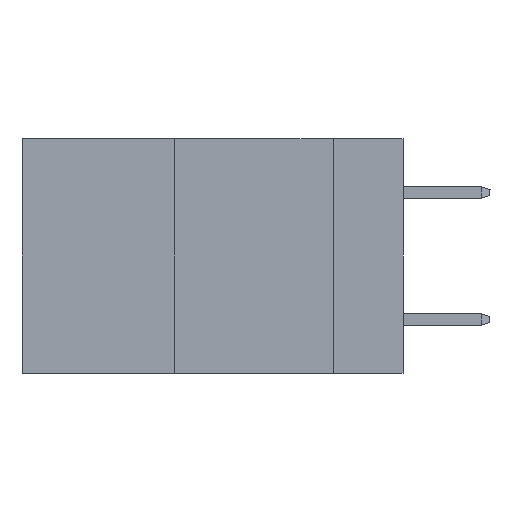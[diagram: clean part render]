
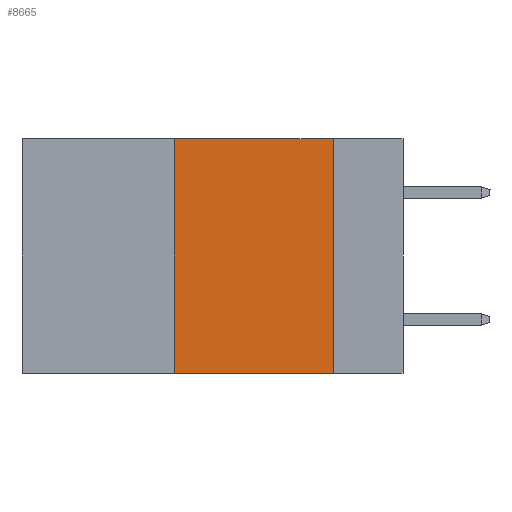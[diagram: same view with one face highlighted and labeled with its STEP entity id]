
A CAD part, left-side view. The second image highlights one B-rep face of the part: STEP entity #8665.
In plain terms, the highlighted planar face has unit normal (-1, 0, 0).
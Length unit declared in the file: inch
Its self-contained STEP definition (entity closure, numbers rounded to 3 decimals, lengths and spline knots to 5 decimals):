
#156 = VECTOR ( 'NONE', #3510, 39.37008 ) ;
#412 = DIRECTION ( 'NONE',  ( 0., 0., -1. ) ) ;
#846 = ORIENTED_EDGE ( 'NONE', *, *, #11870, .F. ) ;
#1116 = LINE ( 'NONE', #7848, #8153 ) ;
#1615 = CARTESIAN_POINT ( 'NONE',  ( 0., 0.11, -0.37 ) ) ;
#2389 = FACE_OUTER_BOUND ( 'NONE', #6721, .T. ) ;
#2730 = ORIENTED_EDGE ( 'NONE', *, *, #11583, .T. ) ;
#2786 = DIRECTION ( 'NONE',  ( 0., 0., -1. ) ) ;
#2893 = CARTESIAN_POINT ( 'NONE',  ( 0., 0.6, 0. ) ) ;
#3047 = DIRECTION ( 'NONE',  ( 0., -1., 0. ) ) ;
#3251 = DIRECTION ( 'NONE',  ( 0., 0., 1. ) ) ;
#3368 = ORIENTED_EDGE ( 'NONE', *, *, #9267, .F. ) ;
#3478 = AXIS2_PLACEMENT_3D ( 'NONE', #2893, #10849, #412 ) ;
#3487 = VECTOR ( 'NONE', #2786, 39.37008 ) ;
#3510 = DIRECTION ( 'NONE',  ( 0., -1., 0. ) ) ;
#4015 = CARTESIAN_POINT ( 'NONE',  ( 0., 0.36, 0. ) ) ;
#4054 = VERTEX_POINT ( 'NONE', #10416 ) ;
#5623 = CARTESIAN_POINT ( 'NONE',  ( 0., 0.36, -0.37 ) ) ;
#5711 = VECTOR ( 'NONE', #3251, 39.37008 ) ;
#6721 = EDGE_LOOP ( 'NONE', ( #9879, #846, #3368, #2730 ) ) ;
#7492 = VERTEX_POINT ( 'NONE', #4015 ) ;
#7846 = VERTEX_POINT ( 'NONE', #5623 ) ;
#7848 = CARTESIAN_POINT ( 'NONE',  ( 0., 0.6, 0. ) ) ;
#7867 = CARTESIAN_POINT ( 'NONE',  ( 0., 0.36, 0. ) ) ;
#8153 = VECTOR ( 'NONE', #3047, 39.37008 ) ;
#8497 = VERTEX_POINT ( 'NONE', #1615 ) ;
#8665 = ADVANCED_FACE ( 'NONE', ( #2389 ), #8690, .F. ) ;
#8690 = PLANE ( 'NONE',  #3478 ) ;
#8913 = EDGE_CURVE ( 'NONE', #4054, #8497, #11378, .T. ) ;
#9139 = LINE ( 'NONE', #12112, #156 ) ;
#9267 = EDGE_CURVE ( 'NONE', #7846, #7492, #10787, .T. ) ;
#9481 = CARTESIAN_POINT ( 'NONE',  ( 0., 0.11, 0. ) ) ;
#9879 = ORIENTED_EDGE ( 'NONE', *, *, #8913, .F. ) ;
#10416 = CARTESIAN_POINT ( 'NONE',  ( 0., 0.11, 0. ) ) ;
#10787 = LINE ( 'NONE', #7867, #5711 ) ;
#10849 = DIRECTION ( 'NONE',  ( 1., 0., 0. ) ) ;
#11378 = LINE ( 'NONE', #9481, #3487 ) ;
#11583 = EDGE_CURVE ( 'NONE', #7846, #8497, #9139, .T. ) ;
#11870 = EDGE_CURVE ( 'NONE', #7492, #4054, #1116, .T. ) ;
#12112 = CARTESIAN_POINT ( 'NONE',  ( 0., 0.6, -0.37 ) ) ;
